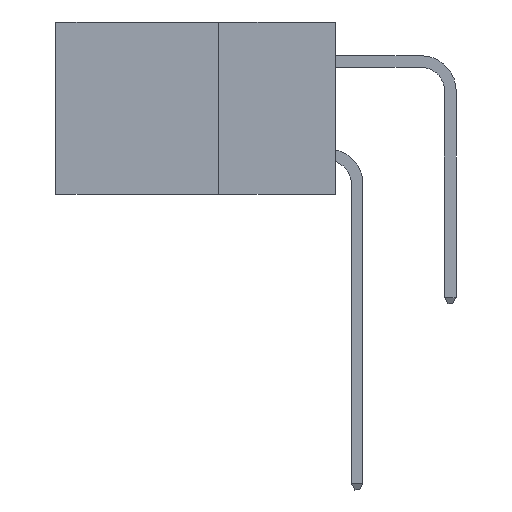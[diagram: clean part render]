
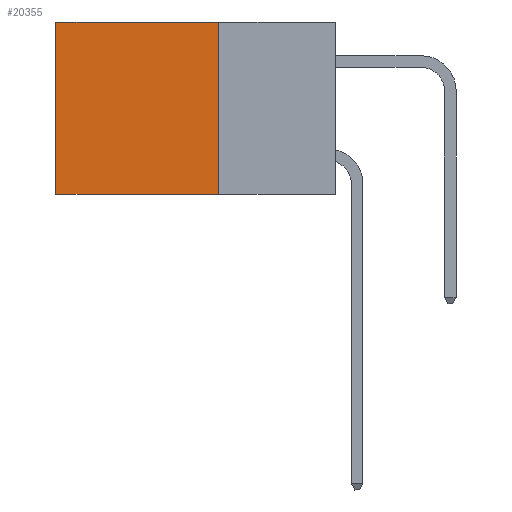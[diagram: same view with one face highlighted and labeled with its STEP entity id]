
A CAD part, left-side view. The second image highlights one B-rep face of the part: STEP entity #20355.
In plain terms, the highlighted planar face has unit normal (-1, 0, 0).
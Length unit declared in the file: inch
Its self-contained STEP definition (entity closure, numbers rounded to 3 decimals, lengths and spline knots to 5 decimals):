
#422 = VERTEX_POINT ( 'NONE', #7939 ) ;
#3285 = AXIS2_PLACEMENT_3D ( 'NONE', #4745, #27730, #8048 ) ;
#4286 = VECTOR ( 'NONE', #9616, 39.37008 ) ;
#4745 = CARTESIAN_POINT ( 'NONE',  ( 0.2875, 0.25, 0. ) ) ;
#5460 = ORIENTED_EDGE ( 'NONE', *, *, #9301, .F. ) ;
#6791 = CARTESIAN_POINT ( 'NONE',  ( 0.2875, 0.25, 0. ) ) ;
#7548 = VECTOR ( 'NONE', #13289, 39.37008 ) ;
#7939 = CARTESIAN_POINT ( 'NONE',  ( 0.2875, 0.6, 0. ) ) ;
#8048 = DIRECTION ( 'NONE',  ( 0., 0., -1. ) ) ;
#8227 = CARTESIAN_POINT ( 'NONE',  ( 0.2875, 0.25, -0.37 ) ) ;
#8939 = VECTOR ( 'NONE', #22309, 39.37008 ) ;
#9301 = EDGE_CURVE ( 'NONE', #29210, #21008, #23345, .T. ) ;
#9616 = DIRECTION ( 'NONE',  ( 0., 1., 0. ) ) ;
#9756 = CARTESIAN_POINT ( 'NONE',  ( 0.2875, 0.25, 0. ) ) ;
#12603 = EDGE_CURVE ( 'NONE', #422, #21008, #38933, .T. ) ;
#13289 = DIRECTION ( 'NONE',  ( 0., 0., -1. ) ) ;
#13321 = VECTOR ( 'NONE', #30610, 39.37008 ) ;
#14504 = FACE_OUTER_BOUND ( 'NONE', #32560, .T. ) ;
#15687 = EDGE_CURVE ( 'NONE', #33455, #422, #35055, .T. ) ;
#16257 = LINE ( 'NONE', #32513, #7548 ) ;
#20190 = ORIENTED_EDGE ( 'NONE', *, *, #24264, .F. ) ;
#20265 = ORIENTED_EDGE ( 'NONE', *, *, #12603, .T. ) ;
#20355 = ADVANCED_FACE ( 'NONE', ( #14504 ), #41001, .F. ) ;
#21008 = VERTEX_POINT ( 'NONE', #28347 ) ;
#22261 = ORIENTED_EDGE ( 'NONE', *, *, #15687, .T. ) ;
#22309 = DIRECTION ( 'NONE',  ( 0., 1., 0. ) ) ;
#23345 = LINE ( 'NONE', #32066, #8939 ) ;
#24264 = EDGE_CURVE ( 'NONE', #33455, #29210, #16257, .T. ) ;
#27730 = DIRECTION ( 'NONE',  ( 1., 0., 0. ) ) ;
#28347 = CARTESIAN_POINT ( 'NONE',  ( 0.2875, 0.6, -0.37 ) ) ;
#29210 = VERTEX_POINT ( 'NONE', #8227 ) ;
#30610 = DIRECTION ( 'NONE',  ( 0., 0., -1. ) ) ;
#32066 = CARTESIAN_POINT ( 'NONE',  ( 0.2875, 0.25, -0.37 ) ) ;
#32513 = CARTESIAN_POINT ( 'NONE',  ( 0.2875, 0.25, 0. ) ) ;
#32560 = EDGE_LOOP ( 'NONE', ( #20265, #5460, #20190, #22261 ) ) ;
#33455 = VERTEX_POINT ( 'NONE', #6791 ) ;
#35055 = LINE ( 'NONE', #9756, #4286 ) ;
#37590 = CARTESIAN_POINT ( 'NONE',  ( 0.2875, 0.6, 0. ) ) ;
#38933 = LINE ( 'NONE', #37590, #13321 ) ;
#41001 = PLANE ( 'NONE',  #3285 ) ;
